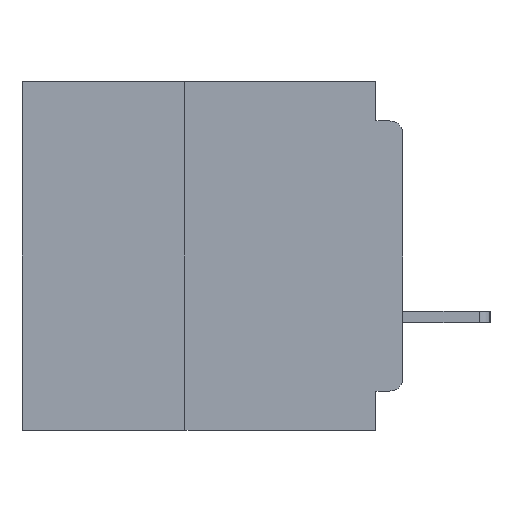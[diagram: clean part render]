
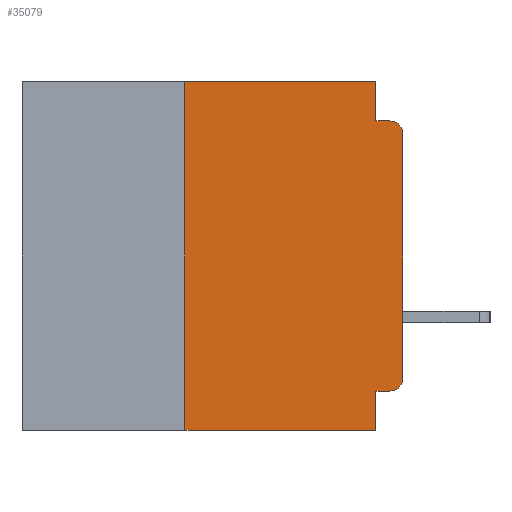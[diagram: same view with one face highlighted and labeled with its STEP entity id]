
A CAD part, left-side view. The second image highlights one B-rep face of the part: STEP entity #35079.
In plain terms, the highlighted planar face has unit normal (-1, 0, 0).
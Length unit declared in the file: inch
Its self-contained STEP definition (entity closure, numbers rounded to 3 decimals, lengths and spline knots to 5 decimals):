
#365 = CARTESIAN_POINT ( 'NONE',  ( 0., 0.031, -0.4 ) ) ;
#613 = CARTESIAN_POINT ( 'NONE',  ( 0., 0.437, 0. ) ) ;
#1367 = CARTESIAN_POINT ( 'NONE',  ( 0., 0.031, 0. ) ) ;
#1415 = VECTOR ( 'NONE', #17848, 39.37008 ) ;
#2041 = LINE ( 'NONE', #53017, #60248 ) ;
#2240 = VERTEX_POINT ( 'NONE', #45669 ) ;
#3899 = VERTEX_POINT ( 'NONE', #47080 ) ;
#4247 = ORIENTED_EDGE ( 'NONE', *, *, #29474, .F. ) ;
#4476 = CARTESIAN_POINT ( 'NONE',  ( 0., 0.015, -0.045 ) ) ;
#5399 = CARTESIAN_POINT ( 'NONE',  ( 0., 0.015, -0.34 ) ) ;
#5403 = DIRECTION ( 'NONE',  ( 0., 0., 1. ) ) ;
#5550 = FACE_OUTER_BOUND ( 'NONE', #52600, .T. ) ;
#5940 = ORIENTED_EDGE ( 'NONE', *, *, #21809, .F. ) ;
#6969 = VERTEX_POINT ( 'NONE', #50574 ) ;
#9185 = CARTESIAN_POINT ( 'NONE',  ( 0., 0., -0.355 ) ) ;
#9716 = LINE ( 'NONE', #21414, #33442 ) ;
#9915 = ORIENTED_EDGE ( 'NONE', *, *, #41041, .T. ) ;
#10147 = DIRECTION ( 'NONE',  ( 0., 0., -1. ) ) ;
#11196 = VECTOR ( 'NONE', #46935, 39.37008 ) ;
#11846 = CARTESIAN_POINT ( 'NONE',  ( 0., 0.031, -0.355 ) ) ;
#11975 = VECTOR ( 'NONE', #5403, 39.37008 ) ;
#12161 = CARTESIAN_POINT ( 'NONE',  ( 0., 0.015, -0.355 ) ) ;
#12512 = EDGE_CURVE ( 'NONE', #3899, #42755, #50104, .T. ) ;
#12535 = CARTESIAN_POINT ( 'NONE',  ( 0., 0., -0.34 ) ) ;
#13066 = CARTESIAN_POINT ( 'NONE',  ( 0., 0., -0.045 ) ) ;
#13270 = VECTOR ( 'NONE', #38276, 39.37008 ) ;
#13595 = ORIENTED_EDGE ( 'NONE', *, *, #42652, .T. ) ;
#14018 = VECTOR ( 'NONE', #48616, 39.37008 ) ;
#15153 = DIRECTION ( 'NONE',  ( 0., 0., -1. ) ) ;
#15773 = VERTEX_POINT ( 'NONE', #12535 ) ;
#16325 = VERTEX_POINT ( 'NONE', #11846 ) ;
#16964 = ORIENTED_EDGE ( 'NONE', *, *, #29246, .F. ) ;
#16985 = AXIS2_PLACEMENT_3D ( 'NONE', #5399, #38495, #10147 ) ;
#17848 = DIRECTION ( 'NONE',  ( 0., -1., 0. ) ) ;
#17858 = ORIENTED_EDGE ( 'NONE', *, *, #60730, .T. ) ;
#19200 = ORIENTED_EDGE ( 'NONE', *, *, #48637, .T. ) ;
#19553 = PLANE ( 'NONE',  #31368 ) ;
#19987 = ORIENTED_EDGE ( 'NONE', *, *, #12512, .F. ) ;
#21414 = CARTESIAN_POINT ( 'NONE',  ( 0., 0.437, 0. ) ) ;
#21809 = EDGE_CURVE ( 'NONE', #6969, #27119, #2041, .T. ) ;
#21816 = CARTESIAN_POINT ( 'NONE',  ( 0., 0.437, -0.4 ) ) ;
#23279 = DIRECTION ( 'NONE',  ( -1., 0., 0. ) ) ;
#26126 = DIRECTION ( 'NONE',  ( 0., -1., 0. ) ) ;
#26652 = CARTESIAN_POINT ( 'NONE',  ( 0., 0.031, -0.4 ) ) ;
#27119 = VERTEX_POINT ( 'NONE', #29986 ) ;
#27996 = ORIENTED_EDGE ( 'NONE', *, *, #53985, .F. ) ;
#29095 = CIRCLE ( 'NONE', #16985, 0.015 ) ;
#29246 = EDGE_CURVE ( 'NONE', #42755, #51155, #51615, .T. ) ;
#29474 = EDGE_CURVE ( 'NONE', #16325, #56440, #41316, .T. ) ;
#29595 = DIRECTION ( 'NONE',  ( 0., 0., 1. ) ) ;
#29986 = CARTESIAN_POINT ( 'NONE',  ( 0., 0.25, 0. ) ) ;
#30185 = VECTOR ( 'NONE', #49911, 39.37008 ) ;
#31368 = AXIS2_PLACEMENT_3D ( 'NONE', #613, #43361, #15153 ) ;
#31552 = AXIS2_PLACEMENT_3D ( 'NONE', #51384, #23279, #56073 ) ;
#33442 = VECTOR ( 'NONE', #26126, 39.37008 ) ;
#34901 = LINE ( 'NONE', #9185, #11196 ) ;
#35079 = ADVANCED_FACE ( 'NONE', ( #5550 ), #19553, .F. ) ;
#35927 = VERTEX_POINT ( 'NONE', #12161 ) ;
#36947 = CIRCLE ( 'NONE', #31552, 0.015 ) ;
#37126 = LINE ( 'NONE', #43151, #11975 ) ;
#38276 = DIRECTION ( 'NONE',  ( 0., 0., -1. ) ) ;
#38495 = DIRECTION ( 'NONE',  ( -1., 0., 0. ) ) ;
#38759 = ORIENTED_EDGE ( 'NONE', *, *, #46818, .F. ) ;
#41041 = EDGE_CURVE ( 'NONE', #35927, #15773, #29095, .T. ) ;
#41316 = LINE ( 'NONE', #365, #13270 ) ;
#42652 = EDGE_CURVE ( 'NONE', #15773, #2240, #37126, .T. ) ;
#42755 = VERTEX_POINT ( 'NONE', #48667 ) ;
#43151 = CARTESIAN_POINT ( 'NONE',  ( 0., 0., 0. ) ) ;
#43361 = DIRECTION ( 'NONE',  ( 1., 0., 0. ) ) ;
#45669 = CARTESIAN_POINT ( 'NONE',  ( 0., 0., -0.06 ) ) ;
#46818 = EDGE_CURVE ( 'NONE', #35927, #16325, #34901, .T. ) ;
#46935 = DIRECTION ( 'NONE',  ( 0., 1., 0. ) ) ;
#47080 = CARTESIAN_POINT ( 'NONE',  ( 0., 0.031, 0. ) ) ;
#48616 = DIRECTION ( 'NONE',  ( 0., 0., -1. ) ) ;
#48637 = EDGE_CURVE ( 'NONE', #6969, #56440, #53700, .T. ) ;
#48667 = CARTESIAN_POINT ( 'NONE',  ( 0., 0.031, -0.045 ) ) ;
#49911 = DIRECTION ( 'NONE',  ( 0., -1., 0. ) ) ;
#50104 = LINE ( 'NONE', #1367, #14018 ) ;
#50574 = CARTESIAN_POINT ( 'NONE',  ( 0., 0.25, -0.4 ) ) ;
#51155 = VERTEX_POINT ( 'NONE', #4476 ) ;
#51384 = CARTESIAN_POINT ( 'NONE',  ( 0., 0.015, -0.06 ) ) ;
#51615 = LINE ( 'NONE', #13066, #1415 ) ;
#52600 = EDGE_LOOP ( 'NONE', ( #13595, #17858, #16964, #19987, #27996, #5940, #19200, #4247, #38759, #9915 ) ) ;
#53017 = CARTESIAN_POINT ( 'NONE',  ( 0., 0.25, -0.4 ) ) ;
#53700 = LINE ( 'NONE', #21816, #30185 ) ;
#53985 = EDGE_CURVE ( 'NONE', #27119, #3899, #9716, .T. ) ;
#56073 = DIRECTION ( 'NONE',  ( 0., 0., -1. ) ) ;
#56440 = VERTEX_POINT ( 'NONE', #26652 ) ;
#60248 = VECTOR ( 'NONE', #29595, 39.37008 ) ;
#60730 = EDGE_CURVE ( 'NONE', #2240, #51155, #36947, .T. ) ;
